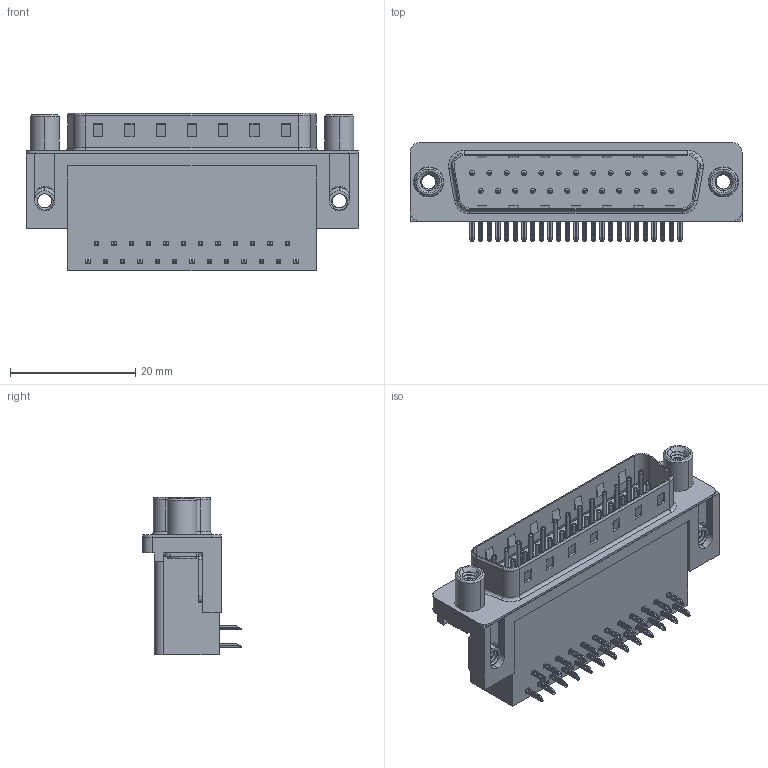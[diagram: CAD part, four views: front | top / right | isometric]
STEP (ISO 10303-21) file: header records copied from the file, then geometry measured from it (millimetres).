
FILE_DESCRIPTION (( 'STEP AP203' ), '1' );
FILE_NAME ('625-025-262-050.STEP', '2018-11-06T01:26:10', ( '' ), ( '' ), 'SwSTEP 2.0', 'SolidWorks 2016', '' );
FILE_SCHEMA (( 'CONFIG_CONTROL_DESIGN' ));
Length unit declared in the file: millimetre
Products named in the file (7): 625 Contact Top; 625 4-40 Threaded Board Mount; 625 Round Threaded Standoff; 625-025-262-050; 625 Housing_25 Socket; 625 Shell_25 Socket; 625 Contact Bottom
Assembly tree (31 placements, depth 2):
  625-025-262-050
    625 Housing_25 Socket
    625 Shell_25 Socket
    625 Contact Bottom  x12
    625 Contact Top  x13
    625 4-40 Threaded Board Mount  x2
    625 Round Threaded Standoff  x2
Bounding box: 53.04 x 15.73 x 25.16 mm (x, y, z)
Volume: 9265.8 mm3; surface area: 9140.2 mm2
Topology: 31 solids, 31 shells, 2291 faces, 5699 edges, 3527 vertices
Faces by surface type: plane 1399, cylinder 681, torus 177, bspline 22, cone 12
Entity records: 24683 total; most frequent: CARTESIAN_POINT 6889, DIRECTION 3417, ORIENTED_EDGE 3362, EDGE_CURVE 1681, VECTOR 1153, LINE 1153, AXIS2_PLACEMENT_3D 1132, VERTEX_POINT 1081
